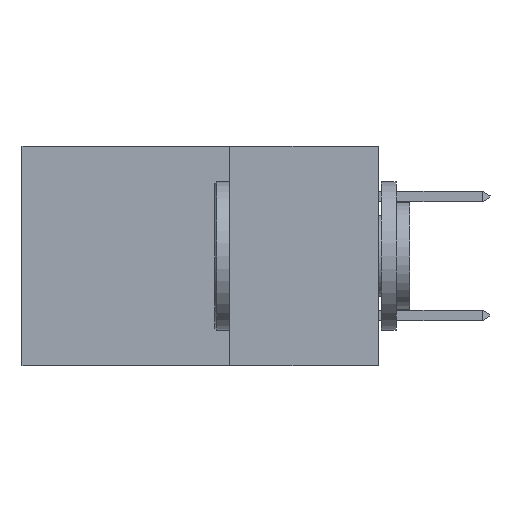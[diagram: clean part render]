
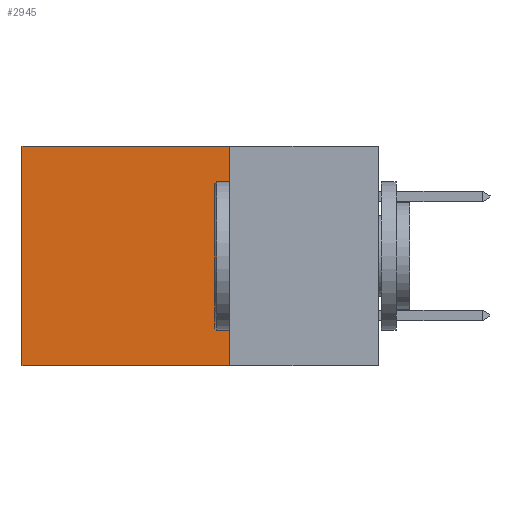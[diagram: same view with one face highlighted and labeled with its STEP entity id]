
A CAD part, left-side view. The second image highlights one B-rep face of the part: STEP entity #2945.
In plain terms, the highlighted planar face has unit normal (-1, 0, 0).
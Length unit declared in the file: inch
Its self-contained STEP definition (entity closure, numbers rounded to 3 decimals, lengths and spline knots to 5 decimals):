
#600 = DIRECTION ( 'NONE',  ( 0., 0., -1. ) ) ;
#903 = VERTEX_POINT ( 'NONE', #8952 ) ;
#1086 = ORIENTED_EDGE ( 'NONE', *, *, #3599, .T. ) ;
#1170 = VECTOR ( 'NONE', #17091, 39.37008 ) ;
#1944 = ORIENTED_EDGE ( 'NONE', *, *, #6475, .F. ) ;
#2558 = EDGE_CURVE ( 'NONE', #903, #14318, #2944, .T. ) ;
#2781 = CARTESIAN_POINT ( 'NONE',  ( 0.2615, 0.25, -0.37 ) ) ;
#2844 = CARTESIAN_POINT ( 'NONE',  ( 0.2615, 0.6, 0. ) ) ;
#2944 = LINE ( 'NONE', #3134, #5026 ) ;
#2945 = ADVANCED_FACE ( 'NONE', ( #5562 ), #11304, .F. ) ;
#3134 = CARTESIAN_POINT ( 'NONE',  ( 0.2615, 0.25, 0. ) ) ;
#3163 = LINE ( 'NONE', #11367, #1170 ) ;
#3599 = EDGE_CURVE ( 'NONE', #14318, #12209, #3163, .T. ) ;
#4088 = EDGE_LOOP ( 'NONE', ( #1086, #7865, #1944, #6356 ) ) ;
#5026 = VECTOR ( 'NONE', #17148, 39.37008 ) ;
#5108 = EDGE_CURVE ( 'NONE', #16418, #12209, #6331, .T. ) ;
#5444 = VECTOR ( 'NONE', #12267, 39.37008 ) ;
#5562 = FACE_OUTER_BOUND ( 'NONE', #4088, .T. ) ;
#6120 = VECTOR ( 'NONE', #600, 39.37008 ) ;
#6331 = LINE ( 'NONE', #8129, #5444 ) ;
#6356 = ORIENTED_EDGE ( 'NONE', *, *, #2558, .T. ) ;
#6475 = EDGE_CURVE ( 'NONE', #903, #16418, #13485, .T. ) ;
#7755 = CARTESIAN_POINT ( 'NONE',  ( 0.2615, 0.25, -0.37 ) ) ;
#7865 = ORIENTED_EDGE ( 'NONE', *, *, #5108, .F. ) ;
#8129 = CARTESIAN_POINT ( 'NONE',  ( 0.2615, 0.25, -0.37 ) ) ;
#8952 = CARTESIAN_POINT ( 'NONE',  ( 0.2615, 0.25, 0. ) ) ;
#11291 = CARTESIAN_POINT ( 'NONE',  ( 0.2615, 0.6, -0.37 ) ) ;
#11304 = PLANE ( 'NONE',  #17342 ) ;
#11367 = CARTESIAN_POINT ( 'NONE',  ( 0.2615, 0.6, -0.37 ) ) ;
#12209 = VERTEX_POINT ( 'NONE', #11291 ) ;
#12267 = DIRECTION ( 'NONE',  ( 0., 1., 0. ) ) ;
#13170 = DIRECTION ( 'NONE',  ( 1., 0., 0. ) ) ;
#13485 = LINE ( 'NONE', #7755, #6120 ) ;
#14318 = VERTEX_POINT ( 'NONE', #2844 ) ;
#16079 = CARTESIAN_POINT ( 'NONE',  ( 0.2615, 0.25, -0.37 ) ) ;
#16174 = DIRECTION ( 'NONE',  ( 0., 0., -1. ) ) ;
#16418 = VERTEX_POINT ( 'NONE', #2781 ) ;
#17091 = DIRECTION ( 'NONE',  ( 0., 0., -1. ) ) ;
#17148 = DIRECTION ( 'NONE',  ( 0., 1., 0. ) ) ;
#17342 = AXIS2_PLACEMENT_3D ( 'NONE', #16079, #13170, #16174 ) ;
